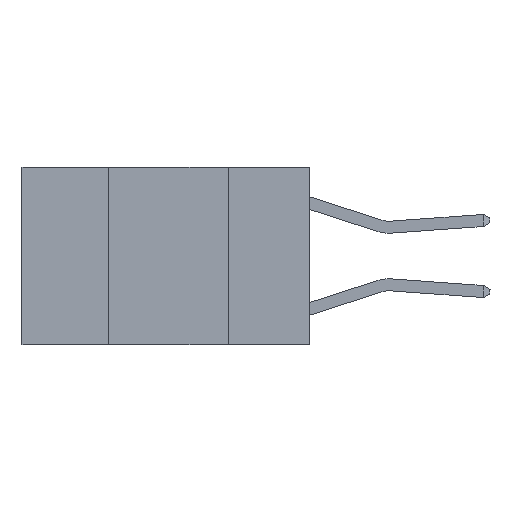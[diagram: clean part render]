
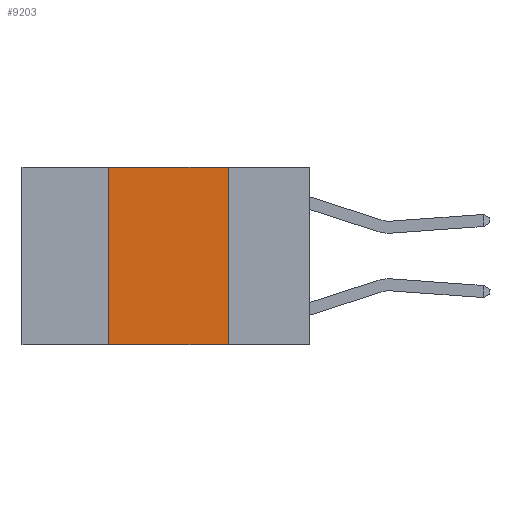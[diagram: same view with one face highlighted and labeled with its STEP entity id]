
A CAD part, left-side view. The second image highlights one B-rep face of the part: STEP entity #9203.
In plain terms, the highlighted planar face has unit normal (-1, 0, 0).
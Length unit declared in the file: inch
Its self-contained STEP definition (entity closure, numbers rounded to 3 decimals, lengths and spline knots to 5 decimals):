
#138 = DIRECTION ( 'NONE',  ( 0., -1., 0. ) ) ;
#202 = VERTEX_POINT ( 'NONE', #774 ) ;
#306 = PLANE ( 'NONE',  #633 ) ;
#523 = VECTOR ( 'NONE', #9318, 39.37008 ) ;
#633 = AXIS2_PLACEMENT_3D ( 'NONE', #9574, #2763, #8087 ) ;
#659 = LINE ( 'NONE', #5639, #4634 ) ;
#774 = CARTESIAN_POINT ( 'NONE',  ( 0., 0.42, 0. ) ) ;
#900 = ORIENTED_EDGE ( 'NONE', *, *, #2600, .F. ) ;
#1355 = ORIENTED_EDGE ( 'NONE', *, *, #2813, .F. ) ;
#1782 = VERTEX_POINT ( 'NONE', #7354 ) ;
#2600 = EDGE_CURVE ( 'NONE', #6584, #1782, #2704, .T. ) ;
#2704 = LINE ( 'NONE', #6751, #6503 ) ;
#2763 = DIRECTION ( 'NONE',  ( 1., 0., 0. ) ) ;
#2813 = EDGE_CURVE ( 'NONE', #202, #6584, #659, .T. ) ;
#2958 = ORIENTED_EDGE ( 'NONE', *, *, #6544, .F. ) ;
#3131 = DIRECTION ( 'NONE',  ( 0., -1., 0. ) ) ;
#3556 = VECTOR ( 'NONE', #3131, 39.37008 ) ;
#4461 = EDGE_LOOP ( 'NONE', ( #900, #1355, #2958, #5793 ) ) ;
#4634 = VECTOR ( 'NONE', #138, 39.37008 ) ;
#4763 = CARTESIAN_POINT ( 'NONE',  ( 0., 0.42, 0. ) ) ;
#5639 = CARTESIAN_POINT ( 'NONE',  ( 0., 0.6, 0. ) ) ;
#5793 = ORIENTED_EDGE ( 'NONE', *, *, #7772, .T. ) ;
#6278 = CARTESIAN_POINT ( 'NONE',  ( 0., 0.42, -0.37 ) ) ;
#6503 = VECTOR ( 'NONE', #7568, 39.37008 ) ;
#6544 = EDGE_CURVE ( 'NONE', #8491, #202, #8787, .T. ) ;
#6584 = VERTEX_POINT ( 'NONE', #9373 ) ;
#6751 = CARTESIAN_POINT ( 'NONE',  ( 0., 0.17, 0. ) ) ;
#6898 = CARTESIAN_POINT ( 'NONE',  ( 0., 0.6, -0.37 ) ) ;
#7354 = CARTESIAN_POINT ( 'NONE',  ( 0., 0.17, -0.37 ) ) ;
#7568 = DIRECTION ( 'NONE',  ( 0., 0., -1. ) ) ;
#7772 = EDGE_CURVE ( 'NONE', #8491, #1782, #9583, .T. ) ;
#8087 = DIRECTION ( 'NONE',  ( 0., 0., -1. ) ) ;
#8491 = VERTEX_POINT ( 'NONE', #6278 ) ;
#8787 = LINE ( 'NONE', #4763, #523 ) ;
#8872 = FACE_OUTER_BOUND ( 'NONE', #4461, .T. ) ;
#9203 = ADVANCED_FACE ( 'NONE', ( #8872 ), #306, .F. ) ;
#9318 = DIRECTION ( 'NONE',  ( 0., 0., 1. ) ) ;
#9373 = CARTESIAN_POINT ( 'NONE',  ( 0., 0.17, 0. ) ) ;
#9574 = CARTESIAN_POINT ( 'NONE',  ( 0., 0.6, 0. ) ) ;
#9583 = LINE ( 'NONE', #6898, #3556 ) ;
